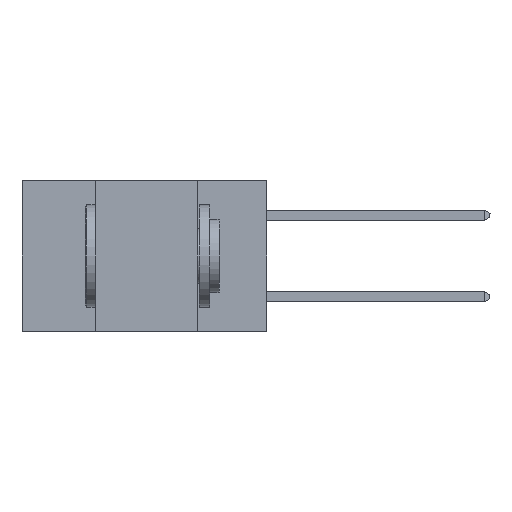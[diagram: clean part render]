
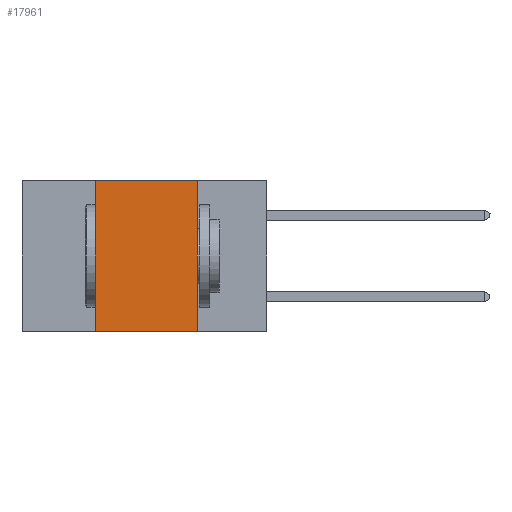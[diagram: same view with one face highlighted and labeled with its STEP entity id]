
A CAD part, left-side view. The second image highlights one B-rep face of the part: STEP entity #17961.
In plain terms, the highlighted planar face has unit normal (-1, 0, 0).
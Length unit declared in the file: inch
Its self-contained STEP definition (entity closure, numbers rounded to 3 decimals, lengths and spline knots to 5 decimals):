
#566 = CARTESIAN_POINT ( 'NONE',  ( 0., 0.6, 0. ) ) ;
#1547 = LINE ( 'NONE', #10452, #14016 ) ;
#3007 = FACE_OUTER_BOUND ( 'NONE', #15925, .T. ) ;
#3512 = CARTESIAN_POINT ( 'NONE',  ( 0., 0.17, 0. ) ) ;
#3585 = DIRECTION ( 'NONE',  ( 0., -1., 0. ) ) ;
#4217 = ORIENTED_EDGE ( 'NONE', *, *, #20854, .F. ) ;
#4519 = ORIENTED_EDGE ( 'NONE', *, *, #11707, .F. ) ;
#4578 = VECTOR ( 'NONE', #16031, 39.37008 ) ;
#5138 = VERTEX_POINT ( 'NONE', #19151 ) ;
#5761 = DIRECTION ( 'NONE',  ( 0., 0., -1. ) ) ;
#6825 = CARTESIAN_POINT ( 'NONE',  ( 0., 0.6, -0.37 ) ) ;
#7165 = ORIENTED_EDGE ( 'NONE', *, *, #21490, .F. ) ;
#9589 = LINE ( 'NONE', #6825, #15445 ) ;
#9835 = CARTESIAN_POINT ( 'NONE',  ( 0., 0.42, 0. ) ) ;
#9858 = VERTEX_POINT ( 'NONE', #3512 ) ;
#10452 = CARTESIAN_POINT ( 'NONE',  ( 0., 0.17, 0. ) ) ;
#11707 = EDGE_CURVE ( 'NONE', #16768, #9858, #20981, .T. ) ;
#12178 = DIRECTION ( 'NONE',  ( 0., 0., -1. ) ) ;
#12470 = CARTESIAN_POINT ( 'NONE',  ( 0., 0.42, 0. ) ) ;
#12676 = ORIENTED_EDGE ( 'NONE', *, *, #14578, .T. ) ;
#14016 = VECTOR ( 'NONE', #12178, 39.37008 ) ;
#14193 = LINE ( 'NONE', #12470, #4578 ) ;
#14578 = EDGE_CURVE ( 'NONE', #20699, #5138, #9589, .T. ) ;
#15445 = VECTOR ( 'NONE', #3585, 39.37008 ) ;
#15925 = EDGE_LOOP ( 'NONE', ( #4217, #4519, #7165, #12676 ) ) ;
#15931 = CARTESIAN_POINT ( 'NONE',  ( 0., 0.6, 0. ) ) ;
#16031 = DIRECTION ( 'NONE',  ( 0., 0., 1. ) ) ;
#16146 = DIRECTION ( 'NONE',  ( 1., 0., 0. ) ) ;
#16164 = DIRECTION ( 'NONE',  ( 0., -1., 0. ) ) ;
#16768 = VERTEX_POINT ( 'NONE', #9835 ) ;
#17961 = ADVANCED_FACE ( 'NONE', ( #3007 ), #19324, .F. ) ;
#18600 = AXIS2_PLACEMENT_3D ( 'NONE', #566, #16146, #5761 ) ;
#19151 = CARTESIAN_POINT ( 'NONE',  ( 0., 0.17, -0.37 ) ) ;
#19324 = PLANE ( 'NONE',  #18600 ) ;
#20045 = CARTESIAN_POINT ( 'NONE',  ( 0., 0.42, -0.37 ) ) ;
#20422 = VECTOR ( 'NONE', #16164, 39.37008 ) ;
#20699 = VERTEX_POINT ( 'NONE', #20045 ) ;
#20854 = EDGE_CURVE ( 'NONE', #9858, #5138, #1547, .T. ) ;
#20981 = LINE ( 'NONE', #15931, #20422 ) ;
#21490 = EDGE_CURVE ( 'NONE', #20699, #16768, #14193, .T. ) ;
